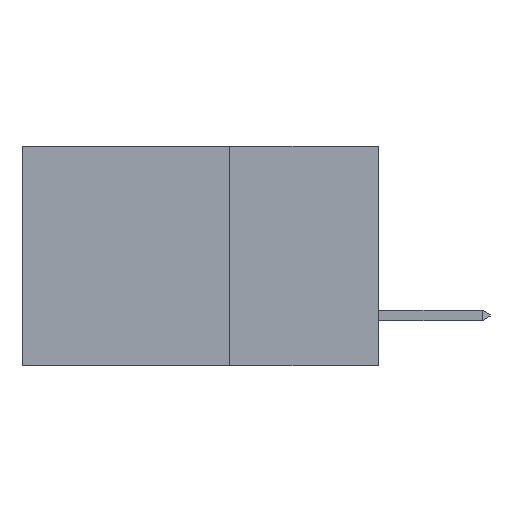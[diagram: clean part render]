
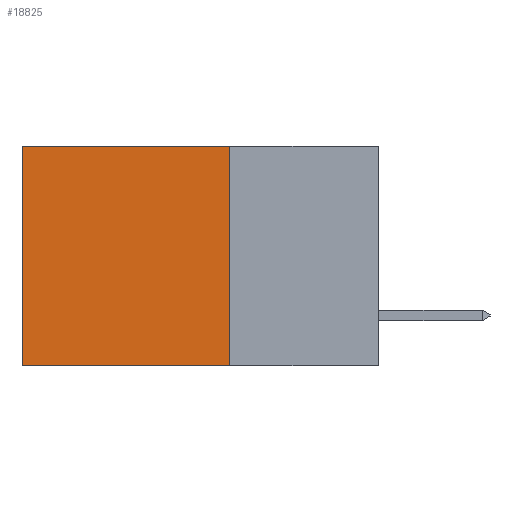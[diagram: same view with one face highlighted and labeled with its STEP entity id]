
A CAD part, left-side view. The second image highlights one B-rep face of the part: STEP entity #18825.
In plain terms, the highlighted planar face has unit normal (-1, 0, 0).
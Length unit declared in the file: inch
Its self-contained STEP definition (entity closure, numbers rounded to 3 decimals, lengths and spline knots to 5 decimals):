
#839 = LINE ( 'NONE', #9060, #14669 ) ;
#2793 = ORIENTED_EDGE ( 'NONE', *, *, #21428, .F. ) ;
#2876 = ORIENTED_EDGE ( 'NONE', *, *, #10360, .F. ) ;
#3379 = CARTESIAN_POINT ( 'NONE',  ( 0.2615, 0.25, -0.37 ) ) ;
#3408 = VECTOR ( 'NONE', #4164, 39.37008 ) ;
#4164 = DIRECTION ( 'NONE',  ( 0., 1., 0. ) ) ;
#4561 = CARTESIAN_POINT ( 'NONE',  ( 0.2615, 0.6, -0.37 ) ) ;
#5449 = CARTESIAN_POINT ( 'NONE',  ( 0.2615, 0.25, 0. ) ) ;
#6031 = CARTESIAN_POINT ( 'NONE',  ( 0.2615, 0.25, -0.37 ) ) ;
#6113 = PLANE ( 'NONE',  #7869 ) ;
#6373 = EDGE_CURVE ( 'NONE', #7525, #11438, #7670, .T. ) ;
#6513 = EDGE_CURVE ( 'NONE', #11438, #14666, #9089, .T. ) ;
#7148 = DIRECTION ( 'NONE',  ( 0., 0., -1. ) ) ;
#7525 = VERTEX_POINT ( 'NONE', #5449 ) ;
#7670 = LINE ( 'NONE', #14890, #3408 ) ;
#7869 = AXIS2_PLACEMENT_3D ( 'NONE', #6031, #18560, #7950 ) ;
#7950 = DIRECTION ( 'NONE',  ( 0., 0., -1. ) ) ;
#8760 = FACE_OUTER_BOUND ( 'NONE', #9025, .T. ) ;
#8913 = CARTESIAN_POINT ( 'NONE',  ( 0.2615, 0.6, -0.37 ) ) ;
#9025 = EDGE_LOOP ( 'NONE', ( #17532, #2876, #2793, #13019 ) ) ;
#9060 = CARTESIAN_POINT ( 'NONE',  ( 0.2615, 0.25, -0.37 ) ) ;
#9089 = LINE ( 'NONE', #4561, #23111 ) ;
#9946 = CARTESIAN_POINT ( 'NONE',  ( 0.2615, 0.25, -0.37 ) ) ;
#10025 = DIRECTION ( 'NONE',  ( 0., 1., 0. ) ) ;
#10360 = EDGE_CURVE ( 'NONE', #19849, #14666, #22454, .T. ) ;
#11438 = VERTEX_POINT ( 'NONE', #19026 ) ;
#13019 = ORIENTED_EDGE ( 'NONE', *, *, #6373, .T. ) ;
#14666 = VERTEX_POINT ( 'NONE', #8913 ) ;
#14669 = VECTOR ( 'NONE', #7148, 39.37008 ) ;
#14890 = CARTESIAN_POINT ( 'NONE',  ( 0.2615, 0.25, 0. ) ) ;
#17000 = DIRECTION ( 'NONE',  ( 0., 0., -1. ) ) ;
#17532 = ORIENTED_EDGE ( 'NONE', *, *, #6513, .T. ) ;
#18560 = DIRECTION ( 'NONE',  ( 1., 0., 0. ) ) ;
#18825 = ADVANCED_FACE ( 'NONE', ( #8760 ), #6113, .F. ) ;
#19026 = CARTESIAN_POINT ( 'NONE',  ( 0.2615, 0.6, 0. ) ) ;
#19849 = VERTEX_POINT ( 'NONE', #3379 ) ;
#21428 = EDGE_CURVE ( 'NONE', #7525, #19849, #839, .T. ) ;
#21914 = VECTOR ( 'NONE', #10025, 39.37008 ) ;
#22454 = LINE ( 'NONE', #9946, #21914 ) ;
#23111 = VECTOR ( 'NONE', #17000, 39.37008 ) ;
